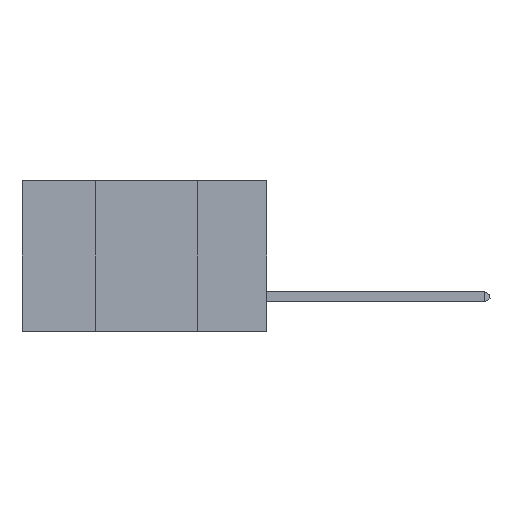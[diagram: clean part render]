
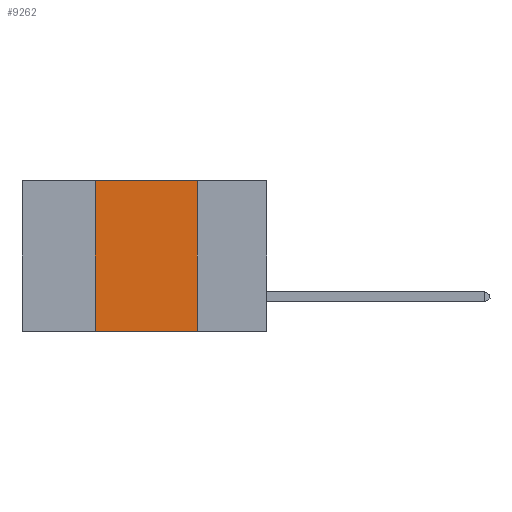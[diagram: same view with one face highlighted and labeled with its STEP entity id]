
A CAD part, left-side view. The second image highlights one B-rep face of the part: STEP entity #9262.
In plain terms, the highlighted planar face has unit normal (-1, 0, 0).
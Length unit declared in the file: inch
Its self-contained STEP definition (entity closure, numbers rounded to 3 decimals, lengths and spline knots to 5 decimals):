
#309 = AXIS2_PLACEMENT_3D ( 'NONE', #17672, #7742, #19360 ) ;
#336 = FACE_OUTER_BOUND ( 'NONE', #8732, .T. ) ;
#339 = CARTESIAN_POINT ( 'NONE',  ( 0., 0.6, 0. ) ) ;
#998 = VECTOR ( 'NONE', #4076, 39.37008 ) ;
#1377 = ORIENTED_EDGE ( 'NONE', *, *, #12723, .F. ) ;
#2633 = VERTEX_POINT ( 'NONE', #6277 ) ;
#4076 = DIRECTION ( 'NONE',  ( 0., 0., 1. ) ) ;
#5698 = VECTOR ( 'NONE', #12170, 39.37008 ) ;
#6057 = PLANE ( 'NONE',  #309 ) ;
#6277 = CARTESIAN_POINT ( 'NONE',  ( 0., 0.42, -0.37 ) ) ;
#7075 = CARTESIAN_POINT ( 'NONE',  ( 0., 0.17, 0. ) ) ;
#7742 = DIRECTION ( 'NONE',  ( 1., 0., 0. ) ) ;
#7842 = CARTESIAN_POINT ( 'NONE',  ( 0., 0.42, 0. ) ) ;
#8163 = CARTESIAN_POINT ( 'NONE',  ( 0., 0.17, 0. ) ) ;
#8732 = EDGE_LOOP ( 'NONE', ( #1377, #17435, #12875, #10718 ) ) ;
#9053 = VERTEX_POINT ( 'NONE', #20730 ) ;
#9262 = ADVANCED_FACE ( 'NONE', ( #336 ), #6057, .F. ) ;
#9817 = EDGE_CURVE ( 'NONE', #2633, #9053, #15090, .T. ) ;
#10718 = ORIENTED_EDGE ( 'NONE', *, *, #9817, .T. ) ;
#11204 = DIRECTION ( 'NONE',  ( 0., -1., 0. ) ) ;
#12170 = DIRECTION ( 'NONE',  ( 0., -1., 0. ) ) ;
#12723 = EDGE_CURVE ( 'NONE', #17475, #9053, #15803, .T. ) ;
#12873 = CARTESIAN_POINT ( 'NONE',  ( 0., 0.6, -0.37 ) ) ;
#12875 = ORIENTED_EDGE ( 'NONE', *, *, #14289, .F. ) ;
#14079 = LINE ( 'NONE', #339, #5698 ) ;
#14289 = EDGE_CURVE ( 'NONE', #2633, #21652, #18331, .T. ) ;
#14595 = VECTOR ( 'NONE', #11204, 39.37008 ) ;
#15090 = LINE ( 'NONE', #12873, #14595 ) ;
#15803 = LINE ( 'NONE', #8163, #19737 ) ;
#17435 = ORIENTED_EDGE ( 'NONE', *, *, #19516, .F. ) ;
#17445 = CARTESIAN_POINT ( 'NONE',  ( 0., 0.42, 0. ) ) ;
#17475 = VERTEX_POINT ( 'NONE', #7075 ) ;
#17672 = CARTESIAN_POINT ( 'NONE',  ( 0., 0.6, 0. ) ) ;
#18331 = LINE ( 'NONE', #17445, #998 ) ;
#19360 = DIRECTION ( 'NONE',  ( 0., 0., -1. ) ) ;
#19516 = EDGE_CURVE ( 'NONE', #21652, #17475, #14079, .T. ) ;
#19737 = VECTOR ( 'NONE', #19793, 39.37008 ) ;
#19793 = DIRECTION ( 'NONE',  ( 0., 0., -1. ) ) ;
#20730 = CARTESIAN_POINT ( 'NONE',  ( 0., 0.17, -0.37 ) ) ;
#21652 = VERTEX_POINT ( 'NONE', #7842 ) ;
